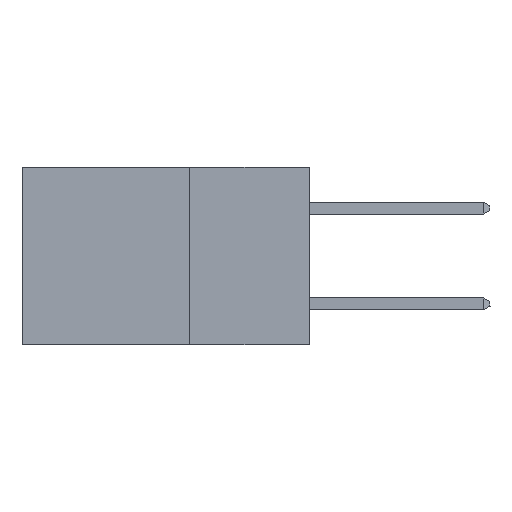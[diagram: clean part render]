
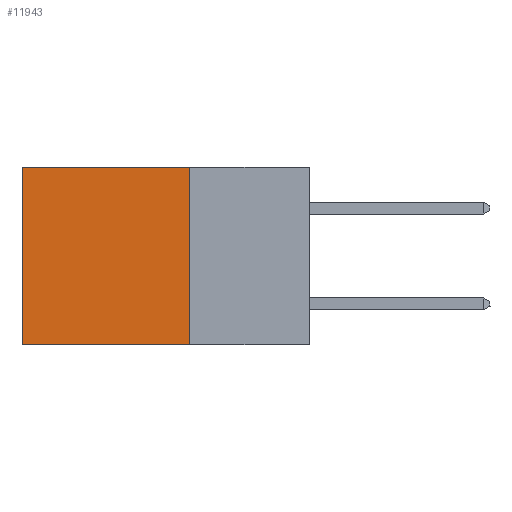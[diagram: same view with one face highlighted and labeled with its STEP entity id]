
A CAD part, left-side view. The second image highlights one B-rep face of the part: STEP entity #11943.
In plain terms, the highlighted planar face has unit normal (-1, 0, 0).
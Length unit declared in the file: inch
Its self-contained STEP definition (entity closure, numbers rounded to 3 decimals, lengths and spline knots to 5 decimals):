
#1666 = AXIS2_PLACEMENT_3D ( 'NONE', #9873, #7882, #20427 ) ;
#2325 = DIRECTION ( 'NONE',  ( 0., 0., -1. ) ) ;
#3332 = DIRECTION ( 'NONE',  ( 0., 0., -1. ) ) ;
#3806 = EDGE_LOOP ( 'NONE', ( #11613, #6847, #18268, #25385 ) ) ;
#3909 = VERTEX_POINT ( 'NONE', #17878 ) ;
#4224 = CARTESIAN_POINT ( 'NONE',  ( 0.2875, 0.25, 0. ) ) ;
#5991 = LINE ( 'NONE', #23805, #23617 ) ;
#6186 = LINE ( 'NONE', #4224, #26760 ) ;
#6847 = ORIENTED_EDGE ( 'NONE', *, *, #23330, .F. ) ;
#6992 = VECTOR ( 'NONE', #3332, 39.37008 ) ;
#7195 = LINE ( 'NONE', #10246, #22500 ) ;
#7703 = CARTESIAN_POINT ( 'NONE',  ( 0.2875, 0.6, 0. ) ) ;
#7747 = CARTESIAN_POINT ( 'NONE',  ( 0.2875, 0.25, 0. ) ) ;
#7882 = DIRECTION ( 'NONE',  ( 1., 0., 0. ) ) ;
#8999 = EDGE_CURVE ( 'NONE', #19759, #11744, #7195, .T. ) ;
#9122 = EDGE_CURVE ( 'NONE', #19759, #3909, #6186, .T. ) ;
#9873 = CARTESIAN_POINT ( 'NONE',  ( 0.2875, 0.25, 0. ) ) ;
#10246 = CARTESIAN_POINT ( 'NONE',  ( 0.2875, 0.25, 0. ) ) ;
#11130 = CARTESIAN_POINT ( 'NONE',  ( 0.2875, 0.6, -0.37 ) ) ;
#11481 = DIRECTION ( 'NONE',  ( 0., 1., 0. ) ) ;
#11613 = ORIENTED_EDGE ( 'NONE', *, *, #26572, .T. ) ;
#11744 = VERTEX_POINT ( 'NONE', #7703 ) ;
#11943 = ADVANCED_FACE ( 'NONE', ( #26974 ), #20701, .F. ) ;
#15142 = LINE ( 'NONE', #25946, #6992 ) ;
#17878 = CARTESIAN_POINT ( 'NONE',  ( 0.2875, 0.25, -0.37 ) ) ;
#18268 = ORIENTED_EDGE ( 'NONE', *, *, #9122, .F. ) ;
#18800 = VERTEX_POINT ( 'NONE', #11130 ) ;
#19759 = VERTEX_POINT ( 'NONE', #7747 ) ;
#20427 = DIRECTION ( 'NONE',  ( 0., 0., -1. ) ) ;
#20701 = PLANE ( 'NONE',  #1666 ) ;
#22500 = VECTOR ( 'NONE', #22560, 39.37008 ) ;
#22560 = DIRECTION ( 'NONE',  ( 0., 1., 0. ) ) ;
#23330 = EDGE_CURVE ( 'NONE', #3909, #18800, #5991, .T. ) ;
#23617 = VECTOR ( 'NONE', #11481, 39.37008 ) ;
#23805 = CARTESIAN_POINT ( 'NONE',  ( 0.2875, 0.25, -0.37 ) ) ;
#25385 = ORIENTED_EDGE ( 'NONE', *, *, #8999, .T. ) ;
#25946 = CARTESIAN_POINT ( 'NONE',  ( 0.2875, 0.6, 0. ) ) ;
#26572 = EDGE_CURVE ( 'NONE', #11744, #18800, #15142, .T. ) ;
#26760 = VECTOR ( 'NONE', #2325, 39.37008 ) ;
#26974 = FACE_OUTER_BOUND ( 'NONE', #3806, .T. ) ;
